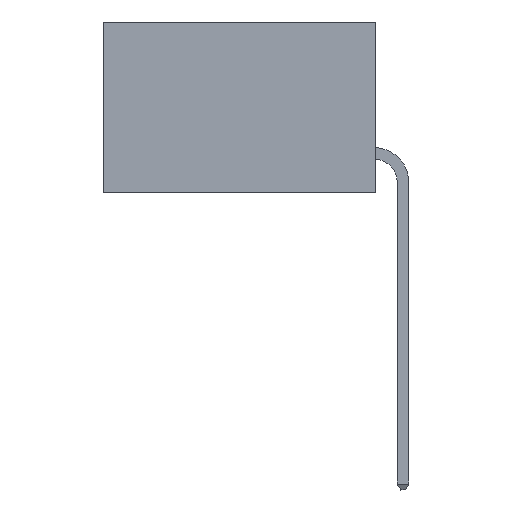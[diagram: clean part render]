
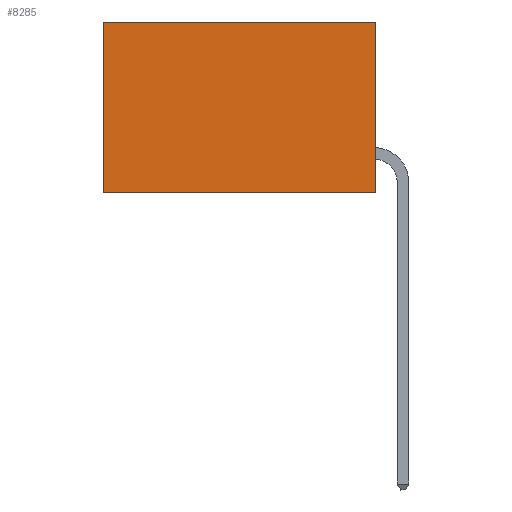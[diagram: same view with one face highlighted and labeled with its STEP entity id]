
A CAD part, left-side view. The second image highlights one B-rep face of the part: STEP entity #8285.
In plain terms, the highlighted planar face has unit normal (-1, 0, 0).
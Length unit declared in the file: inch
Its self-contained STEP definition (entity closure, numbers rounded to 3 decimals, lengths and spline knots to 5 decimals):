
#446 = CARTESIAN_POINT ( 'NONE',  ( 0.277, 0., 0. ) ) ;
#1431 = CARTESIAN_POINT ( 'NONE',  ( 0.277, 0.59, 0. ) ) ;
#1839 = DIRECTION ( 'NONE',  ( 0., 0., -1. ) ) ;
#2395 = CARTESIAN_POINT ( 'NONE',  ( 0.277, 0., -0.37 ) ) ;
#2758 = VERTEX_POINT ( 'NONE', #14901 ) ;
#3272 = LINE ( 'NONE', #9173, #15277 ) ;
#3403 = VECTOR ( 'NONE', #12343, 39.37008 ) ;
#4090 = VERTEX_POINT ( 'NONE', #19072 ) ;
#4618 = CARTESIAN_POINT ( 'NONE',  ( 0.277, 0., -0.37 ) ) ;
#7019 = DIRECTION ( 'NONE',  ( 0., 0., -1. ) ) ;
#7429 = CARTESIAN_POINT ( 'NONE',  ( 0.277, 0.59, -0.37 ) ) ;
#7859 = VERTEX_POINT ( 'NONE', #1431 ) ;
#7995 = ORIENTED_EDGE ( 'NONE', *, *, #18322, .T. ) ;
#8285 = ADVANCED_FACE ( 'NONE', ( #23310 ), #24166, .F. ) ;
#9173 = CARTESIAN_POINT ( 'NONE',  ( 0.277, 0.59, -0.37 ) ) ;
#9521 = ORIENTED_EDGE ( 'NONE', *, *, #22454, .F. ) ;
#9710 = DIRECTION ( 'NONE',  ( 1., 0., 0. ) ) ;
#12285 = AXIS2_PLACEMENT_3D ( 'NONE', #2395, #9710, #26541 ) ;
#12343 = DIRECTION ( 'NONE',  ( 0., 1., 0. ) ) ;
#12700 = EDGE_CURVE ( 'NONE', #4090, #2758, #22739, .T. ) ;
#14901 = CARTESIAN_POINT ( 'NONE',  ( 0.277, 0., -0.37 ) ) ;
#15277 = VECTOR ( 'NONE', #1839, 39.37008 ) ;
#16263 = VECTOR ( 'NONE', #7019, 39.37008 ) ;
#16831 = VERTEX_POINT ( 'NONE', #7429 ) ;
#17367 = DIRECTION ( 'NONE',  ( 0., 1., 0. ) ) ;
#17501 = VECTOR ( 'NONE', #17367, 39.37008 ) ;
#18322 = EDGE_CURVE ( 'NONE', #7859, #16831, #3272, .T. ) ;
#18729 = EDGE_LOOP ( 'NONE', ( #7995, #9521, #21590, #19767 ) ) ;
#19072 = CARTESIAN_POINT ( 'NONE',  ( 0.277, 0., 0. ) ) ;
#19767 = ORIENTED_EDGE ( 'NONE', *, *, #24435, .T. ) ;
#21590 = ORIENTED_EDGE ( 'NONE', *, *, #12700, .F. ) ;
#22454 = EDGE_CURVE ( 'NONE', #2758, #16831, #22648, .T. ) ;
#22648 = LINE ( 'NONE', #24423, #3403 ) ;
#22739 = LINE ( 'NONE', #4618, #16263 ) ;
#23310 = FACE_OUTER_BOUND ( 'NONE', #18729, .T. ) ;
#23941 = LINE ( 'NONE', #446, #17501 ) ;
#24166 = PLANE ( 'NONE',  #12285 ) ;
#24423 = CARTESIAN_POINT ( 'NONE',  ( 0.277, 0., -0.37 ) ) ;
#24435 = EDGE_CURVE ( 'NONE', #4090, #7859, #23941, .T. ) ;
#26541 = DIRECTION ( 'NONE',  ( 0., 0., -1. ) ) ;
